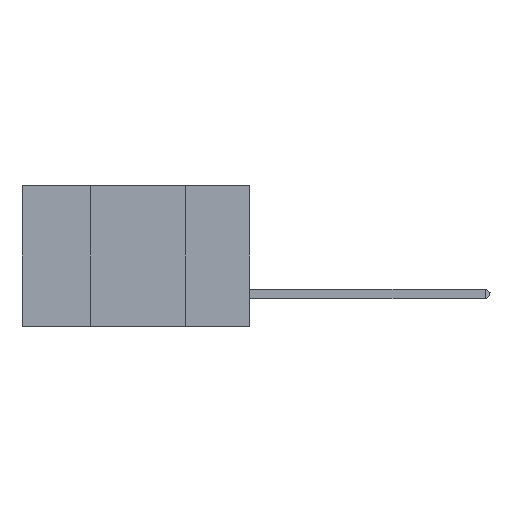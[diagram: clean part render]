
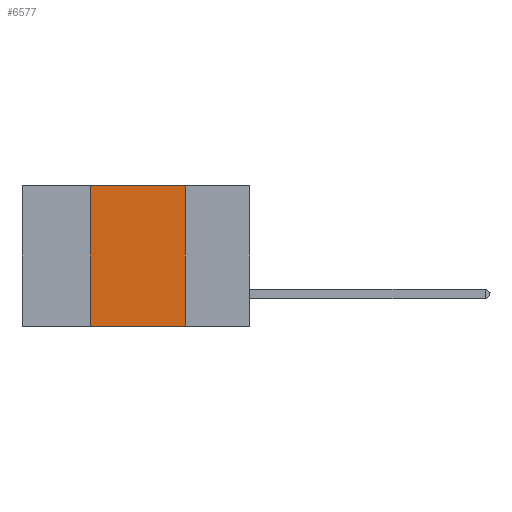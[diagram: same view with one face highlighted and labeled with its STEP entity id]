
A CAD part, left-side view. The second image highlights one B-rep face of the part: STEP entity #6577.
In plain terms, the highlighted planar face has unit normal (-1, 0, 0).
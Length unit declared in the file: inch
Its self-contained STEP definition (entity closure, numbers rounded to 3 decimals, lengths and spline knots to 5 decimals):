
#385 = CARTESIAN_POINT ( 'NONE',  ( 0., 0.6, 0. ) ) ;
#700 = LINE ( 'NONE', #24274, #21604 ) ;
#1161 = VECTOR ( 'NONE', #1346, 39.37008 ) ;
#1346 = DIRECTION ( 'NONE',  ( 0., -1., 0. ) ) ;
#1605 = LINE ( 'NONE', #2299, #16434 ) ;
#2181 = DIRECTION ( 'NONE',  ( 1., 0., 0. ) ) ;
#2299 = CARTESIAN_POINT ( 'NONE',  ( 0., 0.6, 0. ) ) ;
#2448 = DIRECTION ( 'NONE',  ( 0., 0., -1. ) ) ;
#3471 = EDGE_CURVE ( 'NONE', #3547, #12711, #700, .T. ) ;
#3547 = VERTEX_POINT ( 'NONE', #22939 ) ;
#4642 = CARTESIAN_POINT ( 'NONE',  ( 0., 0.42, -0.37 ) ) ;
#6402 = DIRECTION ( 'NONE',  ( 0., -1., 0. ) ) ;
#6468 = EDGE_CURVE ( 'NONE', #9570, #12711, #8101, .T. ) ;
#6473 = LINE ( 'NONE', #24719, #22027 ) ;
#6577 = ADVANCED_FACE ( 'NONE', ( #26150 ), #18338, .F. ) ;
#8101 = LINE ( 'NONE', #15003, #1161 ) ;
#9570 = VERTEX_POINT ( 'NONE', #4642 ) ;
#9748 = EDGE_CURVE ( 'NONE', #20874, #3547, #1605, .T. ) ;
#12711 = VERTEX_POINT ( 'NONE', #26126 ) ;
#14278 = EDGE_CURVE ( 'NONE', #9570, #20874, #6473, .T. ) ;
#15003 = CARTESIAN_POINT ( 'NONE',  ( 0., 0.6, -0.37 ) ) ;
#16046 = AXIS2_PLACEMENT_3D ( 'NONE', #385, #2181, #2448 ) ;
#16434 = VECTOR ( 'NONE', #6402, 39.37008 ) ;
#17162 = ORIENTED_EDGE ( 'NONE', *, *, #6468, .T. ) ;
#17314 = CARTESIAN_POINT ( 'NONE',  ( 0., 0.42, 0. ) ) ;
#18307 = DIRECTION ( 'NONE',  ( 0., 0., -1. ) ) ;
#18338 = PLANE ( 'NONE',  #16046 ) ;
#20318 = ORIENTED_EDGE ( 'NONE', *, *, #14278, .F. ) ;
#20364 = DIRECTION ( 'NONE',  ( 0., 0., 1. ) ) ;
#20874 = VERTEX_POINT ( 'NONE', #17314 ) ;
#21604 = VECTOR ( 'NONE', #18307, 39.37008 ) ;
#22027 = VECTOR ( 'NONE', #20364, 39.37008 ) ;
#22614 = EDGE_LOOP ( 'NONE', ( #23065, #25098, #20318, #17162 ) ) ;
#22939 = CARTESIAN_POINT ( 'NONE',  ( 0., 0.17, 0. ) ) ;
#23065 = ORIENTED_EDGE ( 'NONE', *, *, #3471, .F. ) ;
#24274 = CARTESIAN_POINT ( 'NONE',  ( 0., 0.17, 0. ) ) ;
#24719 = CARTESIAN_POINT ( 'NONE',  ( 0., 0.42, 0. ) ) ;
#25098 = ORIENTED_EDGE ( 'NONE', *, *, #9748, .F. ) ;
#26126 = CARTESIAN_POINT ( 'NONE',  ( 0., 0.17, -0.37 ) ) ;
#26150 = FACE_OUTER_BOUND ( 'NONE', #22614, .T. ) ;
